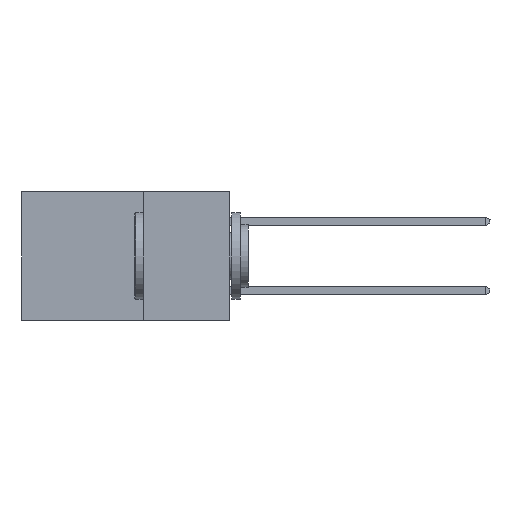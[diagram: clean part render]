
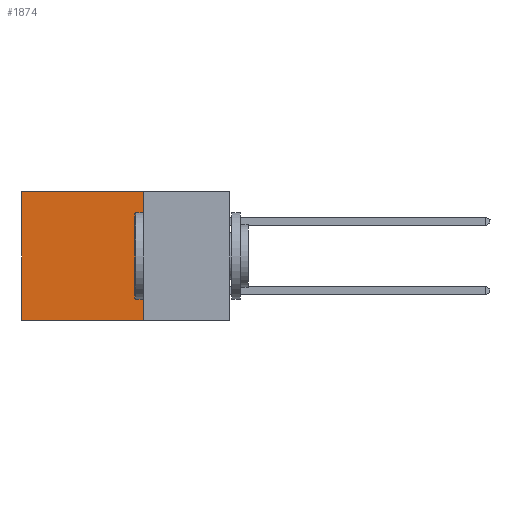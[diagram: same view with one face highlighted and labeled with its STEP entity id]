
A CAD part, left-side view. The second image highlights one B-rep face of the part: STEP entity #1874.
In plain terms, the highlighted planar face has unit normal (-1, 0, 0).
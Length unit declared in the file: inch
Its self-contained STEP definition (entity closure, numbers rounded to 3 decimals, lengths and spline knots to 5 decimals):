
#1310 = ORIENTED_EDGE ( 'NONE', *, *, #6971, .F. ) ;
#1874 = ADVANCED_FACE ( 'NONE', ( #23770 ), #10005, .F. ) ;
#2275 = VERTEX_POINT ( 'NONE', #5597 ) ;
#3309 = EDGE_CURVE ( 'NONE', #2275, #6352, #11957, .T. ) ;
#3560 = VECTOR ( 'NONE', #10275, 39.37008 ) ;
#4244 = LINE ( 'NONE', #9717, #4820 ) ;
#4815 = VECTOR ( 'NONE', #19043, 39.37008 ) ;
#4820 = VECTOR ( 'NONE', #8021, 39.37008 ) ;
#4863 = LINE ( 'NONE', #18786, #4815 ) ;
#5318 = VECTOR ( 'NONE', #24430, 39.37008 ) ;
#5597 = CARTESIAN_POINT ( 'NONE',  ( 0.2615, 0.25, 0. ) ) ;
#5667 = VERTEX_POINT ( 'NONE', #9420 ) ;
#5869 = DIRECTION ( 'NONE',  ( 0., 0., -1. ) ) ;
#6352 = VERTEX_POINT ( 'NONE', #22730 ) ;
#6971 = EDGE_CURVE ( 'NONE', #6352, #17810, #4244, .T. ) ;
#7150 = EDGE_LOOP ( 'NONE', ( #17909, #1310, #12893, #19956 ) ) ;
#8021 = DIRECTION ( 'NONE',  ( 0., 1., 0. ) ) ;
#8200 = CARTESIAN_POINT ( 'NONE',  ( 0.2615, 0.25, -0.37 ) ) ;
#9420 = CARTESIAN_POINT ( 'NONE',  ( 0.2615, 0.6, 0. ) ) ;
#9717 = CARTESIAN_POINT ( 'NONE',  ( 0.2615, 0.25, -0.37 ) ) ;
#10005 = PLANE ( 'NONE',  #15822 ) ;
#10275 = DIRECTION ( 'NONE',  ( 0., 0., -1. ) ) ;
#11957 = LINE ( 'NONE', #8200, #3560 ) ;
#12354 = LINE ( 'NONE', #16537, #5318 ) ;
#12893 = ORIENTED_EDGE ( 'NONE', *, *, #3309, .F. ) ;
#15747 = CARTESIAN_POINT ( 'NONE',  ( 0.2615, 0.25, -0.37 ) ) ;
#15822 = AXIS2_PLACEMENT_3D ( 'NONE', #15747, #23648, #5869 ) ;
#16537 = CARTESIAN_POINT ( 'NONE',  ( 0.2615, 0.6, -0.37 ) ) ;
#17810 = VERTEX_POINT ( 'NONE', #19223 ) ;
#17909 = ORIENTED_EDGE ( 'NONE', *, *, #22227, .T. ) ;
#18786 = CARTESIAN_POINT ( 'NONE',  ( 0.2615, 0.25, 0. ) ) ;
#19043 = DIRECTION ( 'NONE',  ( 0., 1., 0. ) ) ;
#19223 = CARTESIAN_POINT ( 'NONE',  ( 0.2615, 0.6, -0.37 ) ) ;
#19956 = ORIENTED_EDGE ( 'NONE', *, *, #20264, .T. ) ;
#20264 = EDGE_CURVE ( 'NONE', #2275, #5667, #4863, .T. ) ;
#22227 = EDGE_CURVE ( 'NONE', #5667, #17810, #12354, .T. ) ;
#22730 = CARTESIAN_POINT ( 'NONE',  ( 0.2615, 0.25, -0.37 ) ) ;
#23648 = DIRECTION ( 'NONE',  ( 1., 0., 0. ) ) ;
#23770 = FACE_OUTER_BOUND ( 'NONE', #7150, .T. ) ;
#24430 = DIRECTION ( 'NONE',  ( 0., 0., -1. ) ) ;
